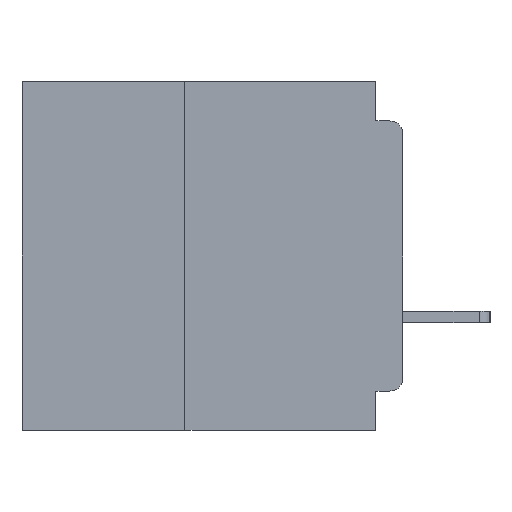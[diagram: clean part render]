
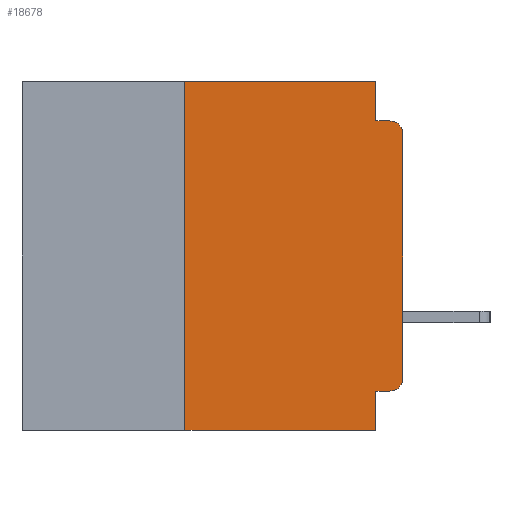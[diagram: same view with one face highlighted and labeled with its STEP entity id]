
A CAD part, left-side view. The second image highlights one B-rep face of the part: STEP entity #18678.
In plain terms, the highlighted planar face has unit normal (-1, 0, 0).
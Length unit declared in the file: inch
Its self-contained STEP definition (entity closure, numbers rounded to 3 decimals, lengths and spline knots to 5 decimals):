
#38 = VERTEX_POINT ( 'NONE', #30318 ) ;
#1043 = ORIENTED_EDGE ( 'NONE', *, *, #32029, .T. ) ;
#2158 = CARTESIAN_POINT ( 'NONE',  ( 0., 0., -0.045 ) ) ;
#3768 = DIRECTION ( 'NONE',  ( 0., 0., -1. ) ) ;
#5675 = VERTEX_POINT ( 'NONE', #18558 ) ;
#7092 = CARTESIAN_POINT ( 'NONE',  ( 0., 0.437, 0. ) ) ;
#8708 = CIRCLE ( 'NONE', #29994, 0.015 ) ;
#9077 = CARTESIAN_POINT ( 'NONE',  ( 0., 0.015, -0.045 ) ) ;
#9203 = VECTOR ( 'NONE', #36962, 39.37008 ) ;
#9260 = VERTEX_POINT ( 'NONE', #26928 ) ;
#9469 = DIRECTION ( 'NONE',  ( 0., -1., 0. ) ) ;
#10818 = VERTEX_POINT ( 'NONE', #9077 ) ;
#10945 = CARTESIAN_POINT ( 'NONE',  ( 0., 0., 0. ) ) ;
#11366 = DIRECTION ( 'NONE',  ( 0., 0., -1. ) ) ;
#11619 = EDGE_CURVE ( 'NONE', #38, #32739, #29545, .T. ) ;
#12363 = CARTESIAN_POINT ( 'NONE',  ( 0., 0.25, -0.4 ) ) ;
#12542 = EDGE_CURVE ( 'NONE', #32739, #10818, #8708, .T. ) ;
#12661 = DIRECTION ( 'NONE',  ( -1., 0., 0. ) ) ;
#13039 = LINE ( 'NONE', #7092, #30402 ) ;
#13160 = VECTOR ( 'NONE', #9469, 39.37008 ) ;
#13611 = VECTOR ( 'NONE', #11366, 39.37008 ) ;
#13657 = CARTESIAN_POINT ( 'NONE',  ( 0., 0.437, -0.4 ) ) ;
#15235 = DIRECTION ( 'NONE',  ( -1., 0., 0. ) ) ;
#16206 = EDGE_CURVE ( 'NONE', #5675, #9260, #13039, .T. ) ;
#16234 = ORIENTED_EDGE ( 'NONE', *, *, #11619, .T. ) ;
#16935 = VERTEX_POINT ( 'NONE', #37162 ) ;
#16981 = ORIENTED_EDGE ( 'NONE', *, *, #12542, .T. ) ;
#17007 = ORIENTED_EDGE ( 'NONE', *, *, #45523, .T. ) ;
#17148 = AXIS2_PLACEMENT_3D ( 'NONE', #22188, #25902, #3768 ) ;
#18558 = CARTESIAN_POINT ( 'NONE',  ( 0., 0.25, 0. ) ) ;
#18678 = ADVANCED_FACE ( 'NONE', ( #35441 ), #44228, .F. ) ;
#19701 = VECTOR ( 'NONE', #25781, 39.37008 ) ;
#20462 = EDGE_LOOP ( 'NONE', ( #16234, #16981, #45350, #44503, #30014, #40615, #1043, #37179, #43286, #17007 ) ) ;
#21812 = LINE ( 'NONE', #34625, #40241 ) ;
#22188 = CARTESIAN_POINT ( 'NONE',  ( 0., 0.437, 0. ) ) ;
#22293 = CARTESIAN_POINT ( 'NONE',  ( 0., 0.031, 0. ) ) ;
#23900 = VERTEX_POINT ( 'NONE', #44431 ) ;
#24466 = VERTEX_POINT ( 'NONE', #24675 ) ;
#24675 = CARTESIAN_POINT ( 'NONE',  ( 0., 0.015, -0.355 ) ) ;
#24915 = EDGE_CURVE ( 'NONE', #24466, #43193, #21812, .T. ) ;
#25781 = DIRECTION ( 'NONE',  ( 0., 0., 1. ) ) ;
#25902 = DIRECTION ( 'NONE',  ( 1., 0., 0. ) ) ;
#26664 = LINE ( 'NONE', #12363, #41581 ) ;
#26802 = VECTOR ( 'NONE', #35741, 39.37008 ) ;
#26928 = CARTESIAN_POINT ( 'NONE',  ( 0., 0.031, 0. ) ) ;
#27026 = EDGE_CURVE ( 'NONE', #43193, #23900, #34376, .T. ) ;
#27987 = LINE ( 'NONE', #13657, #26802 ) ;
#29515 = CARTESIAN_POINT ( 'NONE',  ( 0., 0.25, -0.4 ) ) ;
#29545 = LINE ( 'NONE', #10945, #19701 ) ;
#29994 = AXIS2_PLACEMENT_3D ( 'NONE', #34736, #12661, #38382 ) ;
#30014 = ORIENTED_EDGE ( 'NONE', *, *, #16206, .F. ) ;
#30318 = CARTESIAN_POINT ( 'NONE',  ( 0., 0., -0.34 ) ) ;
#30402 = VECTOR ( 'NONE', #43813, 39.37008 ) ;
#30808 = DIRECTION ( 'NONE',  ( 0., 0., 1. ) ) ;
#32029 = EDGE_CURVE ( 'NONE', #33866, #23900, #27987, .T. ) ;
#32739 = VERTEX_POINT ( 'NONE', #39990 ) ;
#32830 = LINE ( 'NONE', #2158, #13160 ) ;
#33866 = VERTEX_POINT ( 'NONE', #29515 ) ;
#34376 = LINE ( 'NONE', #37156, #13611 ) ;
#34625 = CARTESIAN_POINT ( 'NONE',  ( 0., 0., -0.355 ) ) ;
#34736 = CARTESIAN_POINT ( 'NONE',  ( 0., 0.015, -0.06 ) ) ;
#35441 = FACE_OUTER_BOUND ( 'NONE', #20462, .T. ) ;
#35741 = DIRECTION ( 'NONE',  ( 0., -1., 0. ) ) ;
#36962 = DIRECTION ( 'NONE',  ( 0., 0., -1. ) ) ;
#37156 = CARTESIAN_POINT ( 'NONE',  ( 0., 0.031, -0.4 ) ) ;
#37162 = CARTESIAN_POINT ( 'NONE',  ( 0., 0.031, -0.045 ) ) ;
#37179 = ORIENTED_EDGE ( 'NONE', *, *, #27026, .F. ) ;
#37317 = CARTESIAN_POINT ( 'NONE',  ( 0., 0.015, -0.34 ) ) ;
#37846 = AXIS2_PLACEMENT_3D ( 'NONE', #37317, #15235, #40985 ) ;
#38356 = CARTESIAN_POINT ( 'NONE',  ( 0., 0.031, -0.355 ) ) ;
#38382 = DIRECTION ( 'NONE',  ( 0., 0., -1. ) ) ;
#38572 = LINE ( 'NONE', #22293, #9203 ) ;
#39334 = EDGE_CURVE ( 'NONE', #33866, #5675, #26664, .T. ) ;
#39990 = CARTESIAN_POINT ( 'NONE',  ( 0., 0., -0.06 ) ) ;
#40241 = VECTOR ( 'NONE', #41806, 39.37008 ) ;
#40615 = ORIENTED_EDGE ( 'NONE', *, *, #39334, .F. ) ;
#40985 = DIRECTION ( 'NONE',  ( 0., 0., -1. ) ) ;
#41581 = VECTOR ( 'NONE', #30808, 39.37008 ) ;
#41806 = DIRECTION ( 'NONE',  ( 0., 1., 0. ) ) ;
#42130 = EDGE_CURVE ( 'NONE', #16935, #10818, #32830, .T. ) ;
#43193 = VERTEX_POINT ( 'NONE', #38356 ) ;
#43286 = ORIENTED_EDGE ( 'NONE', *, *, #24915, .F. ) ;
#43813 = DIRECTION ( 'NONE',  ( 0., -1., 0. ) ) ;
#44228 = PLANE ( 'NONE',  #17148 ) ;
#44265 = EDGE_CURVE ( 'NONE', #9260, #16935, #38572, .T. ) ;
#44431 = CARTESIAN_POINT ( 'NONE',  ( 0., 0.031, -0.4 ) ) ;
#44503 = ORIENTED_EDGE ( 'NONE', *, *, #44265, .F. ) ;
#45350 = ORIENTED_EDGE ( 'NONE', *, *, #42130, .F. ) ;
#45523 = EDGE_CURVE ( 'NONE', #24466, #38, #47046, .T. ) ;
#47046 = CIRCLE ( 'NONE', #37846, 0.015 ) ;
